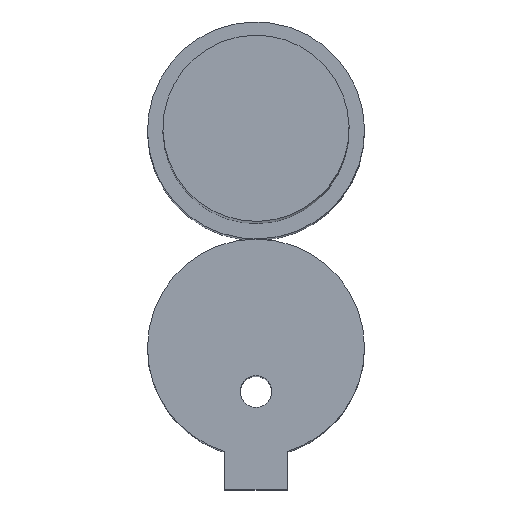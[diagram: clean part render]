
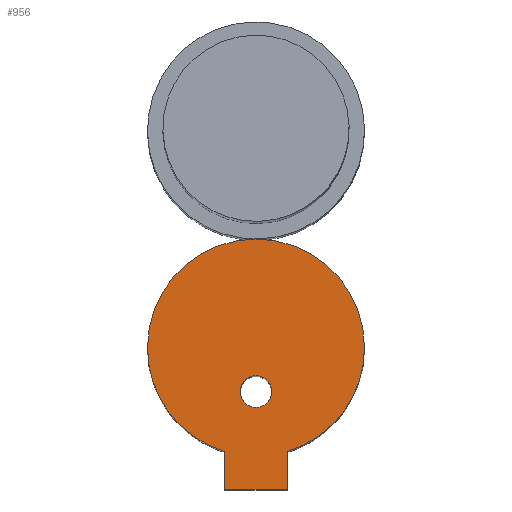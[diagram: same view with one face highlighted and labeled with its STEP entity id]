
A CAD part, top view. The second image highlights one B-rep face of the part: STEP entity #956.
In plain terms, the highlighted planar face has unit normal (0, 0, 1).
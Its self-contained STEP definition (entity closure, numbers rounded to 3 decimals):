
#2 = CARTESIAN_POINT ( 'NONE',  ( -2.75, -12.46, 0. ) ) ;
#10 = DIRECTION ( 'NONE',  ( 0., 0., 1. ) ) ;
#11 = EDGE_CURVE ( 'NONE', #545, #1267, #576, .T. ) ;
#18 = DIRECTION ( 'NONE',  ( 1., 0., 0. ) ) ;
#29 = VECTOR ( 'NONE', #133, 1000. ) ;
#30 = CARTESIAN_POINT ( 'NONE',  ( 2.75, -6.54, 0. ) ) ;
#34 = DIRECTION ( 'NONE',  ( 1., 0., 0. ) ) ;
#76 = EDGE_LOOP ( 'NONE', ( #1154, #1323 ) ) ;
#80 = DIRECTION ( 'NONE',  ( 0., 0., 1. ) ) ;
#94 = AXIS2_PLACEMENT_3D ( 'NONE', #1331, #981, #34 ) ;
#96 = DIRECTION ( 'NONE',  ( 1., 0., 0. ) ) ;
#125 = EDGE_CURVE ( 'NONE', #615, #1251, #353, .T. ) ;
#133 = DIRECTION ( 'NONE',  ( 0., -1., 0. ) ) ;
#160 = CARTESIAN_POINT ( 'NONE',  ( -2.75, -6.54, 0. ) ) ;
#174 = LINE ( 'NONE', #403, #603 ) ;
#186 = FACE_OUTER_BOUND ( 'NONE', #1047, .T. ) ;
#201 = CARTESIAN_POINT ( 'NONE',  ( 0., 0., 0. ) ) ;
#215 = LINE ( 'NONE', #30, #1324 ) ;
#217 = DIRECTION ( 'NONE',  ( 0., 0., 1. ) ) ;
#223 = ORIENTED_EDGE ( 'NONE', *, *, #1059, .F. ) ;
#260 = CARTESIAN_POINT ( 'NONE',  ( 1.384, -3.85, 0. ) ) ;
#264 = EDGE_CURVE ( 'NONE', #1267, #1104, #1015, .T. ) ;
#293 = ORIENTED_EDGE ( 'NONE', *, *, #11, .T. ) ;
#334 = AXIS2_PLACEMENT_3D ( 'NONE', #1120, #80, #381 ) ;
#336 = AXIS2_PLACEMENT_3D ( 'NONE', #1269, #741, #1141 ) ;
#337 = VERTEX_POINT ( 'NONE', #565 ) ;
#353 = CIRCLE ( 'NONE', #534, 1.384 ) ;
#369 = EDGE_CURVE ( 'NONE', #337, #1110, #1075, .T. ) ;
#381 = DIRECTION ( 'NONE',  ( 1., 0., 0. ) ) ;
#403 = CARTESIAN_POINT ( 'NONE',  ( -2.75, -12.46, 0. ) ) ;
#432 = DIRECTION ( 'NONE',  ( 0., -1., 0. ) ) ;
#438 = CARTESIAN_POINT ( 'NONE',  ( -9.5, 0., 0. ) ) ;
#468 = EDGE_CURVE ( 'NONE', #1104, #337, #544, .T. ) ;
#518 = EDGE_CURVE ( 'NONE', #1110, #575, #174, .T. ) ;
#534 = AXIS2_PLACEMENT_3D ( 'NONE', #726, #217, #1062 ) ;
#544 = CIRCLE ( 'NONE', #334, 9.5 ) ;
#545 = VERTEX_POINT ( 'NONE', #817 ) ;
#565 = CARTESIAN_POINT ( 'NONE',  ( -2.75, -9.093, 0. ) ) ;
#575 = VERTEX_POINT ( 'NONE', #641 ) ;
#576 = CIRCLE ( 'NONE', #1337, 9.5 ) ;
#595 = DIRECTION ( 'NONE',  ( 1., 0., 0. ) ) ;
#603 = VECTOR ( 'NONE', #595, 1000. ) ;
#615 = VERTEX_POINT ( 'NONE', #260 ) ;
#641 = CARTESIAN_POINT ( 'NONE',  ( 2.75, -12.46, 0. ) ) ;
#668 = CARTESIAN_POINT ( 'NONE',  ( 9.5, 0., 0. ) ) ;
#686 = AXIS2_PLACEMENT_3D ( 'NONE', #980, #1210, #18 ) ;
#711 = FACE_BOUND ( 'NONE', #76, .T. ) ;
#726 = CARTESIAN_POINT ( 'NONE',  ( 0., -3.85, 0. ) ) ;
#741 = DIRECTION ( 'NONE',  ( 0., 0., 1. ) ) ;
#755 = EDGE_CURVE ( 'NONE', #1251, #615, #1294, .T. ) ;
#817 = CARTESIAN_POINT ( 'NONE',  ( 2.75, -9.093, 0. ) ) ;
#859 = ORIENTED_EDGE ( 'NONE', *, *, #369, .T. ) ;
#871 = CARTESIAN_POINT ( 'NONE',  ( -1.384, -3.85, 0. ) ) ;
#923 = PLANE ( 'NONE',  #336 ) ;
#956 = ADVANCED_FACE ( 'NONE', ( #186, #711 ), #923, .T. ) ;
#980 = CARTESIAN_POINT ( 'NONE',  ( 0., 0., 0. ) ) ;
#981 = DIRECTION ( 'NONE',  ( 0., 0., 1. ) ) ;
#982 = ORIENTED_EDGE ( 'NONE', *, *, #264, .T. ) ;
#1015 = CIRCLE ( 'NONE', #686, 9.5 ) ;
#1047 = EDGE_LOOP ( 'NONE', ( #293, #982, #1052, #859, #1314, #223 ) ) ;
#1052 = ORIENTED_EDGE ( 'NONE', *, *, #468, .T. ) ;
#1059 = EDGE_CURVE ( 'NONE', #545, #575, #215, .T. ) ;
#1062 = DIRECTION ( 'NONE',  ( 1., 0., 0. ) ) ;
#1075 = LINE ( 'NONE', #160, #29 ) ;
#1104 = VERTEX_POINT ( 'NONE', #438 ) ;
#1110 = VERTEX_POINT ( 'NONE', #2 ) ;
#1120 = CARTESIAN_POINT ( 'NONE',  ( 0., 0., 0. ) ) ;
#1141 = DIRECTION ( 'NONE',  ( 1., 0., 0. ) ) ;
#1154 = ORIENTED_EDGE ( 'NONE', *, *, #125, .F. ) ;
#1210 = DIRECTION ( 'NONE',  ( 0., 0., 1. ) ) ;
#1251 = VERTEX_POINT ( 'NONE', #871 ) ;
#1267 = VERTEX_POINT ( 'NONE', #668 ) ;
#1269 = CARTESIAN_POINT ( 'NONE',  ( 0., 0., 0. ) ) ;
#1294 = CIRCLE ( 'NONE', #94, 1.384 ) ;
#1314 = ORIENTED_EDGE ( 'NONE', *, *, #518, .T. ) ;
#1323 = ORIENTED_EDGE ( 'NONE', *, *, #755, .F. ) ;
#1324 = VECTOR ( 'NONE', #432, 1000. ) ;
#1331 = CARTESIAN_POINT ( 'NONE',  ( 0., -3.85, 0. ) ) ;
#1337 = AXIS2_PLACEMENT_3D ( 'NONE', #201, #10, #96 ) ;
